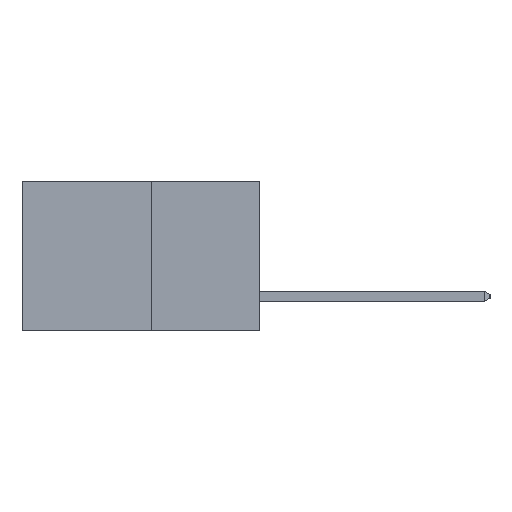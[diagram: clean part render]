
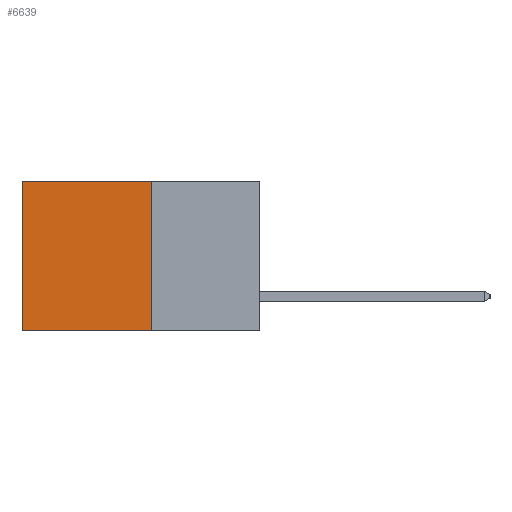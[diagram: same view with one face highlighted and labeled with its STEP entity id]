
A CAD part, left-side view. The second image highlights one B-rep face of the part: STEP entity #6639.
In plain terms, the highlighted planar face has unit normal (-1, 0, 0).
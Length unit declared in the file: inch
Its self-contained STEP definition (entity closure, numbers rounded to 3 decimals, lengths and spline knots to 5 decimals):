
#400 = VECTOR ( 'NONE', #3619, 39.37008 ) ;
#2640 = LINE ( 'NONE', #4608, #23557 ) ;
#2841 = EDGE_CURVE ( 'NONE', #15688, #12849, #6004, .T. ) ;
#3619 = DIRECTION ( 'NONE',  ( 0., 1., 0. ) ) ;
#3864 = EDGE_CURVE ( 'NONE', #25299, #15688, #2640, .T. ) ;
#4608 = CARTESIAN_POINT ( 'NONE',  ( 0.277, 0.27, -0.37 ) ) ;
#4751 = EDGE_LOOP ( 'NONE', ( #9479, #15485, #20457, #19949 ) ) ;
#5705 = CARTESIAN_POINT ( 'NONE',  ( 0.277, 0.59, -0.37 ) ) ;
#6004 = LINE ( 'NONE', #13799, #400 ) ;
#6639 = ADVANCED_FACE ( 'NONE', ( #20101 ), #23161, .F. ) ;
#6948 = LINE ( 'NONE', #5705, #17067 ) ;
#9137 = CARTESIAN_POINT ( 'NONE',  ( 0.277, 0.27, -0.37 ) ) ;
#9479 = ORIENTED_EDGE ( 'NONE', *, *, #15101, .T. ) ;
#12849 = VERTEX_POINT ( 'NONE', #23782 ) ;
#13178 = DIRECTION ( 'NONE',  ( 0., 0., -1. ) ) ;
#13799 = CARTESIAN_POINT ( 'NONE',  ( 0.277, 0.27, -0.37 ) ) ;
#14412 = VECTOR ( 'NONE', #19033, 39.37008 ) ;
#15101 = EDGE_CURVE ( 'NONE', #18823, #12849, #6948, .T. ) ;
#15485 = ORIENTED_EDGE ( 'NONE', *, *, #2841, .F. ) ;
#15688 = VERTEX_POINT ( 'NONE', #16024 ) ;
#16024 = CARTESIAN_POINT ( 'NONE',  ( 0.277, 0.27, -0.37 ) ) ;
#17067 = VECTOR ( 'NONE', #23721, 39.37008 ) ;
#18823 = VERTEX_POINT ( 'NONE', #20521 ) ;
#19033 = DIRECTION ( 'NONE',  ( 0., 1., 0. ) ) ;
#19774 = LINE ( 'NONE', #24899, #14412 ) ;
#19949 = ORIENTED_EDGE ( 'NONE', *, *, #24319, .T. ) ;
#20101 = FACE_OUTER_BOUND ( 'NONE', #4751, .T. ) ;
#20457 = ORIENTED_EDGE ( 'NONE', *, *, #3864, .F. ) ;
#20521 = CARTESIAN_POINT ( 'NONE',  ( 0.277, 0.59, 0. ) ) ;
#22294 = CARTESIAN_POINT ( 'NONE',  ( 0.277, 0.27, 0. ) ) ;
#22770 = DIRECTION ( 'NONE',  ( 0., 0., -1. ) ) ;
#23161 = PLANE ( 'NONE',  #24454 ) ;
#23557 = VECTOR ( 'NONE', #22770, 39.37008 ) ;
#23721 = DIRECTION ( 'NONE',  ( 0., 0., -1. ) ) ;
#23782 = CARTESIAN_POINT ( 'NONE',  ( 0.277, 0.59, -0.37 ) ) ;
#24319 = EDGE_CURVE ( 'NONE', #25299, #18823, #19774, .T. ) ;
#24454 = AXIS2_PLACEMENT_3D ( 'NONE', #9137, #25138, #13178 ) ;
#24899 = CARTESIAN_POINT ( 'NONE',  ( 0.277, 0.27, 0. ) ) ;
#25138 = DIRECTION ( 'NONE',  ( 1., 0., 0. ) ) ;
#25299 = VERTEX_POINT ( 'NONE', #22294 ) ;
